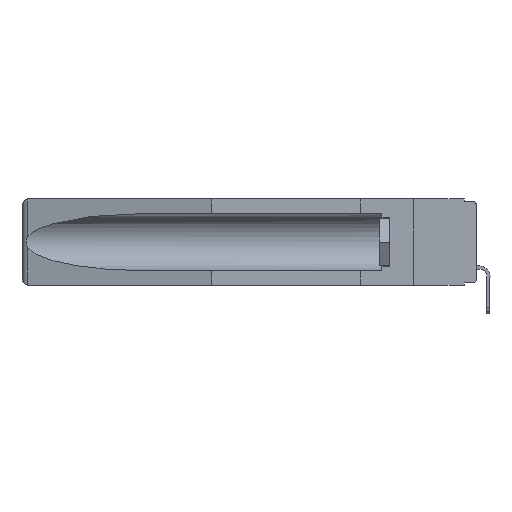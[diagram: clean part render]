
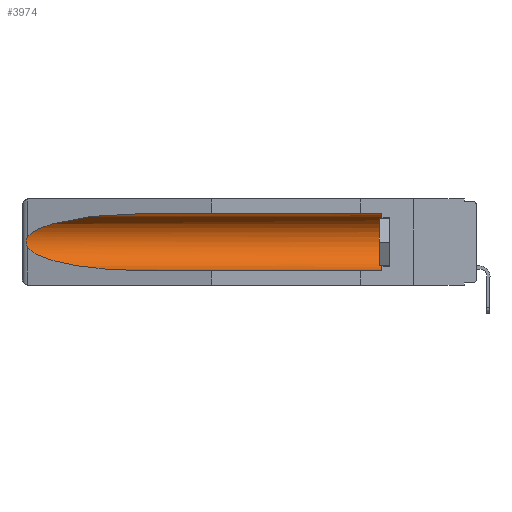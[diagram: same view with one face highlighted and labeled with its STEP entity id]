
A CAD part, left-side view. The second image highlights one B-rep face of the part: STEP entity #3974.
In plain terms, the highlighted cylindrical face has radius 2.857 mm (diameter 5.715 mm), a partial arc.
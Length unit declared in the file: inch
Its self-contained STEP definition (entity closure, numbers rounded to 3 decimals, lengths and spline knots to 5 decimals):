
#980 = EDGE_CURVE ( 'NONE', #1281, #3111, #19852, .T. ) ;
#1281 = VERTEX_POINT ( 'NONE', #10226 ) ;
#1449 = CARTESIAN_POINT ( 'NONE',  ( 0.2675, 1.53308, -0.17534 ) ) ;
#1763 = VERTEX_POINT ( 'NONE', #14435 ) ;
#1974 =( BOUNDED_CURVE ( )  B_SPLINE_CURVE ( 3, ( #20963, #23002, #23175, #15156 ),
 .UNSPECIFIED., .F., .F. ) 
 B_SPLINE_CURVE_WITH_KNOTS ( ( 4, 4 ),
 ( 0.1948, 1.5708 ),
 .UNSPECIFIED. ) 
 CURVE ( )  GEOMETRIC_REPRESENTATION_ITEM ( )  RATIONAL_B_SPLINE_CURVE ( ( 1., 0.848, 0.848, 1. ) ) 
 REPRESENTATION_ITEM ( '' )  );
#1977 = DIRECTION ( 'NONE',  ( 0., 1., 0. ) ) ;
#2446 = FACE_OUTER_BOUND ( 'NONE', #17385, .T. ) ;
#3111 = VERTEX_POINT ( 'NONE', #14670 ) ;
#3357 = CARTESIAN_POINT ( 'NONE',  ( 0.155, 0.126, -0.059 ) ) ;
#3376 = DIRECTION ( 'NONE',  ( 0., 0., 1. ) ) ;
#3502 = ORIENTED_EDGE ( 'NONE', *, *, #9982, .T. ) ;
#3677 = CARTESIAN_POINT ( 'NONE',  ( 0.26597, 1.5296, -0.19026 ) ) ;
#3974 = ADVANCED_FACE ( 'NONE', ( #2446 ), #12605, .F. ) ;
#5133 = CARTESIAN_POINT ( 'NONE',  ( 0.21114, 1.30732, -0.059 ) ) ;
#5312 = CARTESIAN_POINT ( 'NONE',  ( 0.26597, 1.52961, -0.15275 ) ) ;
#5411 = VECTOR ( 'NONE', #5504, 39.37008 ) ;
#5504 = DIRECTION ( 'NONE',  ( 0., 1., 0. ) ) ;
#6971 = LINE ( 'NONE', #16419, #7301 ) ;
#7280 = CARTESIAN_POINT ( 'NONE',  ( 0.2675, 1.53308, -0.16763 ) ) ;
#7301 = VECTOR ( 'NONE', #18286, 39.37008 ) ;
#7365 = CARTESIAN_POINT ( 'NONE',  ( 0.26654, 1.53092, -0.15636 ) ) ;
#8179 = CARTESIAN_POINT ( 'NONE',  ( 0.155, 1.07973, -0.059 ) ) ;
#9034 = CARTESIAN_POINT ( 'NONE',  ( 0.26537, 1.52718, -0.19328 ) ) ;
#9158 = CARTESIAN_POINT ( 'NONE',  ( 0.26537, 1.52718, -0.14972 ) ) ;
#9211 = B_SPLINE_CURVE_WITH_KNOTS ( 'NONE', 3,
 ( #21015, #5312, #7365, #11262, #7280, #1449, #9258, #9432, #3677, #15208 ),
 .UNSPECIFIED., .F., .F.,
 ( 4, 2, 2, 2, 4 ),
 ( 0., 0.00029, 0.00058, 0.00087, 0.00117 ),
 .UNSPECIFIED. ) ;
#9258 = CARTESIAN_POINT ( 'NONE',  ( 0.2673, 1.53269, -0.17917 ) ) ;
#9432 = CARTESIAN_POINT ( 'NONE',  ( 0.26655, 1.53094, -0.18657 ) ) ;
#9695 = ORIENTED_EDGE ( 'NONE', *, *, #16833, .T. ) ;
#9982 = EDGE_CURVE ( 'NONE', #1763, #18446, #9211, .T. ) ;
#10226 = CARTESIAN_POINT ( 'NONE',  ( 0.155, 0.126, -0.284 ) ) ;
#11262 = CARTESIAN_POINT ( 'NONE',  ( 0.2673, 1.5327, -0.16383 ) ) ;
#11661 = EDGE_CURVE ( 'NONE', #1281, #14444, #21428, .T. ) ;
#12605 = CYLINDRICAL_SURFACE ( 'NONE', #21306, 0.1125 ) ;
#13567 = ORIENTED_EDGE ( 'NONE', *, *, #23649, .T. ) ;
#13692 = CARTESIAN_POINT ( 'NONE',  ( 0.155, -0.30754, -0.1715 ) ) ;
#13706 = VERTEX_POINT ( 'NONE', #8179 ) ;
#13789 = ORIENTED_EDGE ( 'NONE', *, *, #18504, .T. ) ;
#14435 = CARTESIAN_POINT ( 'NONE',  ( 0.26537, 1.52718, -0.14972 ) ) ;
#14444 = VERTEX_POINT ( 'NONE', #3357 ) ;
#14670 = CARTESIAN_POINT ( 'NONE',  ( 0.155, 1.07973, -0.284 ) ) ;
#15156 = CARTESIAN_POINT ( 'NONE',  ( 0.155, 1.07973, -0.284 ) ) ;
#15208 = CARTESIAN_POINT ( 'NONE',  ( 0.26537, 1.52718, -0.19328 ) ) ;
#15748 = DIRECTION ( 'NONE',  ( 0., 0., 1. ) ) ;
#16419 = CARTESIAN_POINT ( 'NONE',  ( 0.155, -0.30754, -0.059 ) ) ;
#16833 = EDGE_CURVE ( 'NONE', #13706, #1763, #18665, .T. ) ;
#17385 = EDGE_LOOP ( 'NONE', ( #9695, #3502, #13789, #18658, #18292, #13567 ) ) ;
#18286 = DIRECTION ( 'NONE',  ( 0., 1., 0. ) ) ;
#18292 = ORIENTED_EDGE ( 'NONE', *, *, #11661, .T. ) ;
#18446 = VERTEX_POINT ( 'NONE', #9034 ) ;
#18504 = EDGE_CURVE ( 'NONE', #18446, #3111, #1974, .T. ) ;
#18658 = ORIENTED_EDGE ( 'NONE', *, *, #980, .F. ) ;
#18665 =( BOUNDED_CURVE ( )  B_SPLINE_CURVE ( 3, ( #19198, #5133, #21002, #9158 ),
 .UNSPECIFIED., .F., .F. ) 
 B_SPLINE_CURVE_WITH_KNOTS ( ( 4, 4 ),
 ( 4.71239, 6.08839 ),
 .UNSPECIFIED. ) 
 CURVE ( )  GEOMETRIC_REPRESENTATION_ITEM ( )  RATIONAL_B_SPLINE_CURVE ( ( 1., 0.848, 0.848, 1. ) ) 
 REPRESENTATION_ITEM ( '' )  );
#19198 = CARTESIAN_POINT ( 'NONE',  ( 0.155, 1.07973, -0.059 ) ) ;
#19852 = LINE ( 'NONE', #21037, #5411 ) ;
#20709 = DIRECTION ( 'NONE',  ( 0., -1., 0. ) ) ;
#20963 = CARTESIAN_POINT ( 'NONE',  ( 0.26537, 1.52718, -0.19328 ) ) ;
#21002 = CARTESIAN_POINT ( 'NONE',  ( 0.25451, 1.48313, -0.09465 ) ) ;
#21015 = CARTESIAN_POINT ( 'NONE',  ( 0.26537, 1.52718, -0.14972 ) ) ;
#21037 = CARTESIAN_POINT ( 'NONE',  ( 0.155, -0.30754, -0.284 ) ) ;
#21306 = AXIS2_PLACEMENT_3D ( 'NONE', #13692, #1977, #15748 ) ;
#21428 = CIRCLE ( 'NONE', #23062, 0.1125 ) ;
#22751 = CARTESIAN_POINT ( 'NONE',  ( 0.155, 0.126, -0.1715 ) ) ;
#23002 = CARTESIAN_POINT ( 'NONE',  ( 0.25451, 1.48313, -0.24835 ) ) ;
#23062 = AXIS2_PLACEMENT_3D ( 'NONE', #22751, #20709, #3376 ) ;
#23175 = CARTESIAN_POINT ( 'NONE',  ( 0.21114, 1.30732, -0.284 ) ) ;
#23649 = EDGE_CURVE ( 'NONE', #14444, #13706, #6971, .T. ) ;
